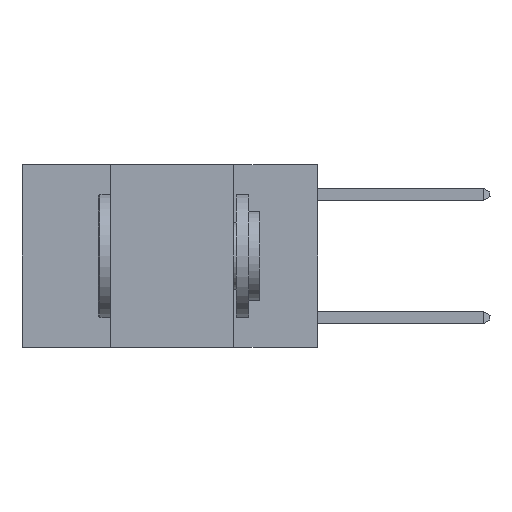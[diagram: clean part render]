
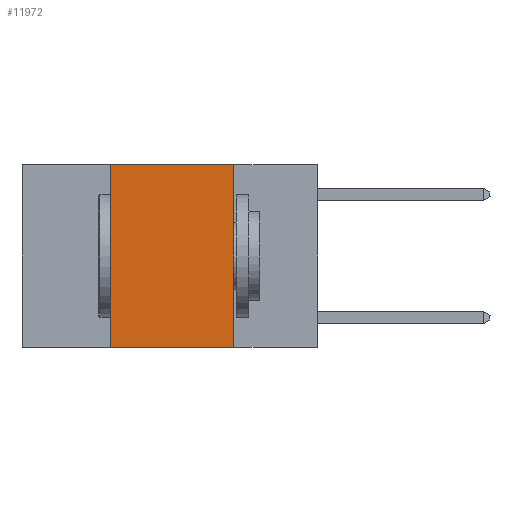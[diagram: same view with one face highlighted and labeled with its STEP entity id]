
A CAD part, left-side view. The second image highlights one B-rep face of the part: STEP entity #11972.
In plain terms, the highlighted planar face has unit normal (-1, 0, 0).
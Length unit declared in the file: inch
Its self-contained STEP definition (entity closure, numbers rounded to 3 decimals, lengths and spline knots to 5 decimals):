
#149 = CARTESIAN_POINT ( 'NONE',  ( 0., 0.42, 0. ) ) ;
#428 = CARTESIAN_POINT ( 'NONE',  ( 0., 0.42, -0.37 ) ) ;
#466 = LINE ( 'NONE', #11478, #5808 ) ;
#1011 = EDGE_CURVE ( 'NONE', #8643, #12228, #4842, .T. ) ;
#1230 = PLANE ( 'NONE',  #3674 ) ;
#2283 = DIRECTION ( 'NONE',  ( 0., 0., -1. ) ) ;
#2636 = EDGE_CURVE ( 'NONE', #11296, #3262, #12741, .T. ) ;
#2998 = CARTESIAN_POINT ( 'NONE',  ( 0., 0.6, 0. ) ) ;
#3139 = EDGE_LOOP ( 'NONE', ( #11388, #6703, #3513, #5327 ) ) ;
#3262 = VERTEX_POINT ( 'NONE', #5677 ) ;
#3295 = CARTESIAN_POINT ( 'NONE',  ( 0., 0.6, 0. ) ) ;
#3513 = ORIENTED_EDGE ( 'NONE', *, *, #4858, .F. ) ;
#3674 = AXIS2_PLACEMENT_3D ( 'NONE', #3295, #8623, #2283 ) ;
#4842 = LINE ( 'NONE', #7536, #12947 ) ;
#4858 = EDGE_CURVE ( 'NONE', #8643, #11296, #11775, .T. ) ;
#5293 = EDGE_CURVE ( 'NONE', #3262, #12228, #466, .T. ) ;
#5327 = ORIENTED_EDGE ( 'NONE', *, *, #1011, .T. ) ;
#5677 = CARTESIAN_POINT ( 'NONE',  ( 0., 0.17, 0. ) ) ;
#5808 = VECTOR ( 'NONE', #11221, 39.37008 ) ;
#6472 = DIRECTION ( 'NONE',  ( 0., -1., 0. ) ) ;
#6583 = FACE_OUTER_BOUND ( 'NONE', #3139, .T. ) ;
#6703 = ORIENTED_EDGE ( 'NONE', *, *, #2636, .F. ) ;
#7129 = CARTESIAN_POINT ( 'NONE',  ( 0., 0.17, -0.37 ) ) ;
#7378 = VECTOR ( 'NONE', #9139, 39.37008 ) ;
#7536 = CARTESIAN_POINT ( 'NONE',  ( 0., 0.6, -0.37 ) ) ;
#8243 = VECTOR ( 'NONE', #11807, 39.37008 ) ;
#8471 = CARTESIAN_POINT ( 'NONE',  ( 0., 0.42, 0. ) ) ;
#8623 = DIRECTION ( 'NONE',  ( 1., 0., 0. ) ) ;
#8643 = VERTEX_POINT ( 'NONE', #428 ) ;
#9139 = DIRECTION ( 'NONE',  ( 0., -1., 0. ) ) ;
#11221 = DIRECTION ( 'NONE',  ( 0., 0., -1. ) ) ;
#11296 = VERTEX_POINT ( 'NONE', #8471 ) ;
#11388 = ORIENTED_EDGE ( 'NONE', *, *, #5293, .F. ) ;
#11478 = CARTESIAN_POINT ( 'NONE',  ( 0., 0.17, 0. ) ) ;
#11775 = LINE ( 'NONE', #149, #8243 ) ;
#11807 = DIRECTION ( 'NONE',  ( 0., 0., 1. ) ) ;
#11972 = ADVANCED_FACE ( 'NONE', ( #6583 ), #1230, .F. ) ;
#12228 = VERTEX_POINT ( 'NONE', #7129 ) ;
#12741 = LINE ( 'NONE', #2998, #7378 ) ;
#12947 = VECTOR ( 'NONE', #6472, 39.37008 ) ;
